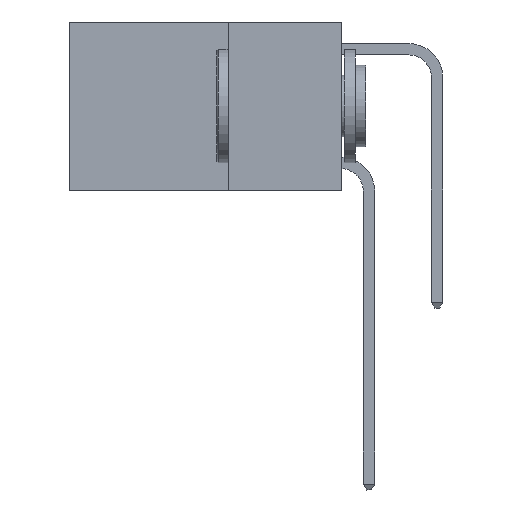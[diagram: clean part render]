
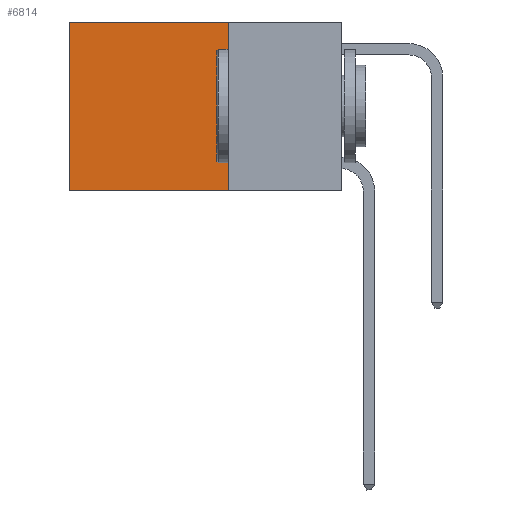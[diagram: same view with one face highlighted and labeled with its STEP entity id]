
A CAD part, left-side view. The second image highlights one B-rep face of the part: STEP entity #6814.
In plain terms, the highlighted planar face has unit normal (-1, 0, 0).
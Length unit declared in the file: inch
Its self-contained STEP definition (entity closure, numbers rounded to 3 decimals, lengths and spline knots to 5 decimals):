
#284 = EDGE_LOOP ( 'NONE', ( #2228, #6512, #11151, #5467 ) ) ;
#427 = LINE ( 'NONE', #10671, #4194 ) ;
#465 = VECTOR ( 'NONE', #9633, 39.37008 ) ;
#475 = AXIS2_PLACEMENT_3D ( 'NONE', #10224, #9196, #7414 ) ;
#1007 = CARTESIAN_POINT ( 'NONE',  ( 0.2625, 0.25, 0. ) ) ;
#1597 = CARTESIAN_POINT ( 'NONE',  ( 0.2625, 0.6, 0. ) ) ;
#2228 = ORIENTED_EDGE ( 'NONE', *, *, #4947, .T. ) ;
#2659 = CARTESIAN_POINT ( 'NONE',  ( 0.2625, 0.25, -0.37 ) ) ;
#3074 = VERTEX_POINT ( 'NONE', #7157 ) ;
#3090 = CARTESIAN_POINT ( 'NONE',  ( 0.2625, 0.25, -0.37 ) ) ;
#3684 = FACE_OUTER_BOUND ( 'NONE', #284, .T. ) ;
#4194 = VECTOR ( 'NONE', #7114, 39.37008 ) ;
#4689 = VERTEX_POINT ( 'NONE', #8205 ) ;
#4817 = LINE ( 'NONE', #1007, #11366 ) ;
#4867 = EDGE_CURVE ( 'NONE', #10080, #3074, #5847, .T. ) ;
#4879 = DIRECTION ( 'NONE',  ( 0., 1., 0. ) ) ;
#4947 = EDGE_CURVE ( 'NONE', #10049, #3074, #8833, .T. ) ;
#5400 = EDGE_CURVE ( 'NONE', #4689, #10080, #427, .T. ) ;
#5467 = ORIENTED_EDGE ( 'NONE', *, *, #8830, .T. ) ;
#5847 = LINE ( 'NONE', #3090, #465 ) ;
#6512 = ORIENTED_EDGE ( 'NONE', *, *, #4867, .F. ) ;
#6814 = ADVANCED_FACE ( 'NONE', ( #3684 ), #11032, .F. ) ;
#7114 = DIRECTION ( 'NONE',  ( 0., 0., -1. ) ) ;
#7129 = VECTOR ( 'NONE', #8772, 39.37008 ) ;
#7157 = CARTESIAN_POINT ( 'NONE',  ( 0.2625, 0.6, -0.37 ) ) ;
#7414 = DIRECTION ( 'NONE',  ( 0., 0., -1. ) ) ;
#8205 = CARTESIAN_POINT ( 'NONE',  ( 0.2625, 0.25, 0. ) ) ;
#8772 = DIRECTION ( 'NONE',  ( 0., 0., -1. ) ) ;
#8830 = EDGE_CURVE ( 'NONE', #4689, #10049, #4817, .T. ) ;
#8833 = LINE ( 'NONE', #8957, #7129 ) ;
#8957 = CARTESIAN_POINT ( 'NONE',  ( 0.2625, 0.6, 0. ) ) ;
#9196 = DIRECTION ( 'NONE',  ( 1., 0., 0. ) ) ;
#9633 = DIRECTION ( 'NONE',  ( 0., 1., 0. ) ) ;
#10049 = VERTEX_POINT ( 'NONE', #1597 ) ;
#10080 = VERTEX_POINT ( 'NONE', #2659 ) ;
#10224 = CARTESIAN_POINT ( 'NONE',  ( 0.2625, 0.25, 0. ) ) ;
#10671 = CARTESIAN_POINT ( 'NONE',  ( 0.2625, 0.25, 0. ) ) ;
#11032 = PLANE ( 'NONE',  #475 ) ;
#11151 = ORIENTED_EDGE ( 'NONE', *, *, #5400, .F. ) ;
#11366 = VECTOR ( 'NONE', #4879, 39.37008 ) ;
